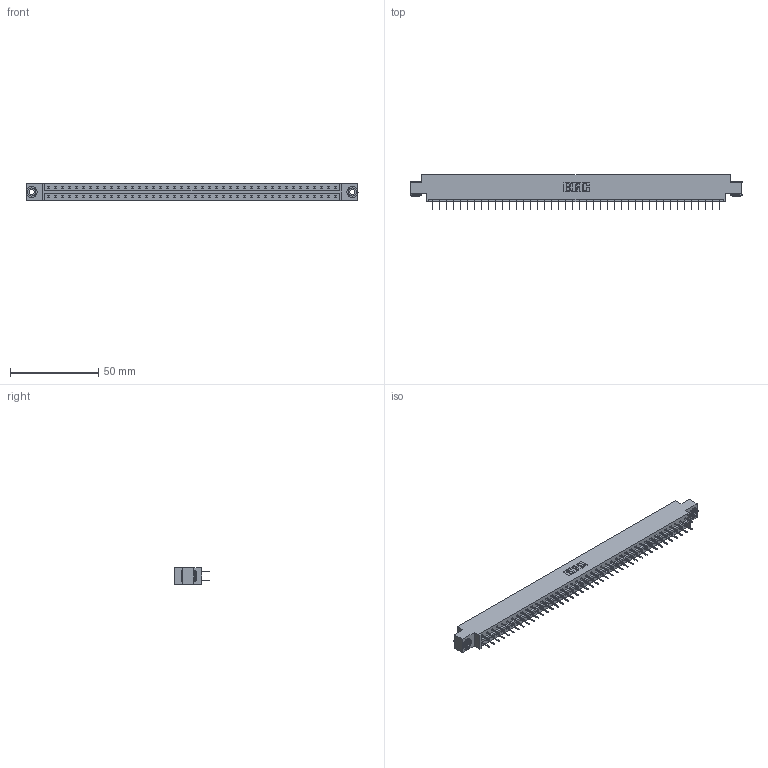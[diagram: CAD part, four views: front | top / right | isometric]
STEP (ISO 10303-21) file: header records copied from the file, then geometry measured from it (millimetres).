
FILE_DESCRIPTION (( 'STEP AP203' ), '1' );
FILE_NAME ('833-084-524-803.STEP', '2020-06-06T01:18:43', ( '' ), ( '' ), 'SwSTEP 2.0', 'SolidWorks 2020', '' );
FILE_SCHEMA (( 'CONFIG_CONTROL_DESIGN' ));
Length unit declared in the file: inch
Products named in the file (4): 833 Part_Offset - .156 Dia - TH; 345-292-001_345-293-124; 833-084-524-803; 345-250-002_345-250-002-102
Assembly tree (87 placements, depth 2):
  833-084-524-803
    833 Part_Offset - .156 Dia - TH
    345-292-001_345-293-124  x84
    345-250-002_345-250-002-102  x2
Bounding box: 187.96 x 19.69 x 9.4 mm (x, y, z)
Volume: 18854.1 mm3; surface area: 22350.5 mm2
Topology: 87 solids, 87 shells, 4860 faces, 13755 edges, 8830 vertices
Faces by surface type: plane 3612, cylinder 1240, cone 8
Entity records: 27876 total; most frequent: CARTESIAN_POINT 4597, ORIENTED_EDGE 4526, DIRECTION 3961, EDGE_CURVE 2263, LINE 2115, VECTOR 2115, VERTEX_POINT 1502, AXIS2_PLACEMENT_3D 923
